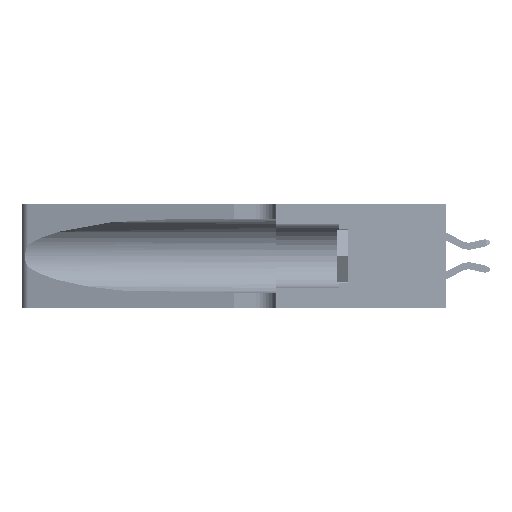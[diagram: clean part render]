
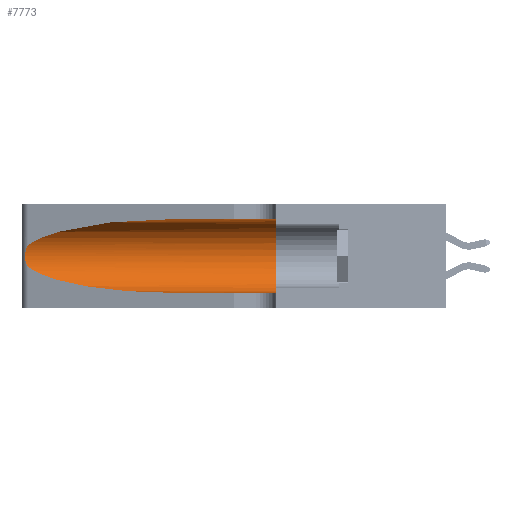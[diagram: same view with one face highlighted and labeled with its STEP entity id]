
A CAD part, left-side view. The second image highlights one B-rep face of the part: STEP entity #7773.
In plain terms, the highlighted cylindrical face has radius 3.308 mm (diameter 6.617 mm), a partial arc.
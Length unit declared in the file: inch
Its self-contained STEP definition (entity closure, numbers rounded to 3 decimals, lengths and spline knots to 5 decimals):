
#312 = EDGE_CURVE ( 'NONE', #32154, #678, #998, .T. ) ;
#678 = VERTEX_POINT ( 'NONE', #14712 ) ;
#725 = LINE ( 'NONE', #29079, #53772 ) ;
#998 =( BOUNDED_CURVE ( )  B_SPLINE_CURVE ( 3, ( #54188, #24978, #33164, #29164 ),
 .UNSPECIFIED., .F., .F. ) 
 B_SPLINE_CURVE_WITH_KNOTS ( ( 4, 4 ),
 ( 1.5708, 2.84003 ),
 .UNSPECIFIED. ) 
 CURVE ( )  GEOMETRIC_REPRESENTATION_ITEM ( )  RATIONAL_B_SPLINE_CURVE ( ( 1., 0.87, 0.87, 1. ) ) 
 REPRESENTATION_ITEM ( '' )  );
#1072 = CARTESIAN_POINT ( 'NONE',  ( 0.1305, 0.35, 0.05475 ) ) ;
#2460 = ORIENTED_EDGE ( 'NONE', *, *, #24936, .T. ) ;
#3120 = DIRECTION ( 'NONE',  ( 0., 0., -1. ) ) ;
#3653 = CARTESIAN_POINT ( 'NONE',  ( 0.18966, 0.96281, 0.05475 ) ) ;
#6674 = EDGE_CURVE ( 'NONE', #678, #36311, #39907, .T. ) ;
#7773 = ADVANCED_FACE ( 'NONE', ( #49015 ), #14359, .F. ) ;
#7824 = CARTESIAN_POINT ( 'NONE',  ( 0.25787, 1.23484, 0.2124 ) ) ;
#9872 = ORIENTED_EDGE ( 'NONE', *, *, #18689, .F. ) ;
#10265 = CARTESIAN_POINT ( 'NONE',  ( 0.1305, 0.72297, 0.05475 ) ) ;
#11420 = VERTEX_POINT ( 'NONE', #10265 ) ;
#11612 = CARTESIAN_POINT ( 'NONE',  ( 0.1305, 1.61858, 0.185 ) ) ;
#11893 = CARTESIAN_POINT ( 'NONE',  ( 0.25487, 1.22718, 0.22369 ) ) ;
#11954 = CARTESIAN_POINT ( 'NONE',  ( 0.2373, 1.15595, 0.08982 ) ) ;
#12067 = CARTESIAN_POINT ( 'NONE',  ( 0.26018, 1.23835, 0.19895 ) ) ;
#12270 = EDGE_LOOP ( 'NONE', ( #12979, #48956, #2460, #24812, #32948, #9872 ) ) ;
#12696 = VECTOR ( 'NONE', #30308, 39.37008 ) ;
#12979 = ORIENTED_EDGE ( 'NONE', *, *, #312, .T. ) ;
#14359 = CYLINDRICAL_SURFACE ( 'NONE', #31501, 0.13025 ) ;
#14712 = CARTESIAN_POINT ( 'NONE',  ( 0.25487, 1.22718, 0.22369 ) ) ;
#16020 = CARTESIAN_POINT ( 'NONE',  ( 0.25487, 1.22718, 0.14631 ) ) ;
#16302 = CARTESIAN_POINT ( 'NONE',  ( 0.26075, 1.23896, 0.178 ) ) ;
#16436 = CARTESIAN_POINT ( 'NONE',  ( 0.1305, 0.72297, 0.31525 ) ) ;
#17312 = VERTEX_POINT ( 'NONE', #47875 ) ;
#18615 = DIRECTION ( 'NONE',  ( 0., 1., 0. ) ) ;
#18689 = EDGE_CURVE ( 'NONE', #32154, #17312, #23864, .T. ) ;
#20530 = CARTESIAN_POINT ( 'NONE',  ( 0.25856, 1.23593, 0.16098 ) ) ;
#21945 = CARTESIAN_POINT ( 'NONE',  ( 0.1305, 1.61858, 0.31525 ) ) ;
#23581 = EDGE_CURVE ( 'NONE', #11420, #30537, #725, .T. ) ;
#23864 = LINE ( 'NONE', #21945, #12696 ) ;
#24556 = CARTESIAN_POINT ( 'NONE',  ( 0.25555, 1.22994, 0.2215 ) ) ;
#24737 = CARTESIAN_POINT ( 'NONE',  ( 0.25639, 1.23186, 0.15144 ) ) ;
#24812 = ORIENTED_EDGE ( 'NONE', *, *, #23581, .T. ) ;
#24936 = EDGE_CURVE ( 'NONE', #36311, #11420, #38221, .T. ) ;
#24978 = CARTESIAN_POINT ( 'NONE',  ( 0.18966, 0.96281, 0.31525 ) ) ;
#26587 = EDGE_CURVE ( 'NONE', #17312, #30537, #46950, .T. ) ;
#28908 = CARTESIAN_POINT ( 'NONE',  ( 0.25487, 1.22718, 0.14631 ) ) ;
#29079 = CARTESIAN_POINT ( 'NONE',  ( 0.1305, 1.61858, 0.05475 ) ) ;
#29164 = CARTESIAN_POINT ( 'NONE',  ( 0.25487, 1.22718, 0.22369 ) ) ;
#30308 = DIRECTION ( 'NONE',  ( 0., -1., 0. ) ) ;
#30537 = VERTEX_POINT ( 'NONE', #1072 ) ;
#31501 = AXIS2_PLACEMENT_3D ( 'NONE', #11612, #53305, #3120 ) ;
#32154 = VERTEX_POINT ( 'NONE', #16436 ) ;
#32908 = CARTESIAN_POINT ( 'NONE',  ( 0.25639, 1.23184, 0.21858 ) ) ;
#32948 = ORIENTED_EDGE ( 'NONE', *, *, #26587, .F. ) ;
#32969 = CARTESIAN_POINT ( 'NONE',  ( 0.1305, 0.72297, 0.05475 ) ) ;
#33164 = CARTESIAN_POINT ( 'NONE',  ( 0.2373, 1.15595, 0.28018 ) ) ;
#34663 = CARTESIAN_POINT ( 'NONE',  ( 0.25487, 1.22718, 0.14631 ) ) ;
#36311 = VERTEX_POINT ( 'NONE', #34663 ) ;
#37085 = CARTESIAN_POINT ( 'NONE',  ( 0.25854, 1.2359, 0.20912 ) ) ;
#38221 =( BOUNDED_CURVE ( )  B_SPLINE_CURVE ( 3, ( #16020, #11954, #3653, #32969 ),
 .UNSPECIFIED., .F., .F. ) 
 B_SPLINE_CURVE_WITH_KNOTS ( ( 4, 4 ),
 ( 3.44316, 4.71239 ),
 .UNSPECIFIED. ) 
 CURVE ( )  GEOMETRIC_REPRESENTATION_ITEM ( )  RATIONAL_B_SPLINE_CURVE ( ( 1., 0.87, 0.87, 1. ) ) 
 REPRESENTATION_ITEM ( '' )  );
#39907 = B_SPLINE_CURVE_WITH_KNOTS ( 'NONE', 3,
 ( #11893, #24556, #32908, #7824, #37085, #12067, #41317, #16302, #45506, #20530, #49729, #24737, #53937, #28908 ),
 .UNSPECIFIED., .F., .F.,
 ( 4, 2, 2, 2, 2, 2, 4 ),
 ( 0., 0.00027, 0.00053, 0.00107, 0.0016, 0.00187, 0.00214 ),
 .UNSPECIFIED. ) ;
#41317 = CARTESIAN_POINT ( 'NONE',  ( 0.26075, 1.23896, 0.19203 ) ) ;
#43587 = CARTESIAN_POINT ( 'NONE',  ( 0.1305, 0.35, 0.185 ) ) ;
#45319 = AXIS2_PLACEMENT_3D ( 'NONE', #43587, #18615, #47814 ) ;
#45506 = CARTESIAN_POINT ( 'NONE',  ( 0.26017, 1.23833, 0.17102 ) ) ;
#46950 = CIRCLE ( 'NONE', #45319, 0.13025 ) ;
#47814 = DIRECTION ( 'NONE',  ( 0., 0., 1. ) ) ;
#47875 = CARTESIAN_POINT ( 'NONE',  ( 0.1305, 0.35, 0.31525 ) ) ;
#48956 = ORIENTED_EDGE ( 'NONE', *, *, #6674, .T. ) ;
#49015 = FACE_OUTER_BOUND ( 'NONE', #12270, .T. ) ;
#49729 = CARTESIAN_POINT ( 'NONE',  ( 0.25789, 1.23486, 0.15765 ) ) ;
#49914 = DIRECTION ( 'NONE',  ( 0., -1., 0. ) ) ;
#53305 = DIRECTION ( 'NONE',  ( 0., -1., 0. ) ) ;
#53772 = VECTOR ( 'NONE', #49914, 39.37008 ) ;
#53937 = CARTESIAN_POINT ( 'NONE',  ( 0.25555, 1.22993, 0.14849 ) ) ;
#54188 = CARTESIAN_POINT ( 'NONE',  ( 0.1305, 0.72297, 0.31525 ) ) ;
